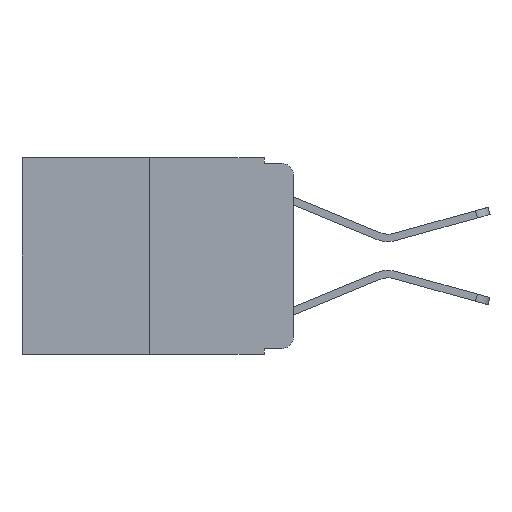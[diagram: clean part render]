
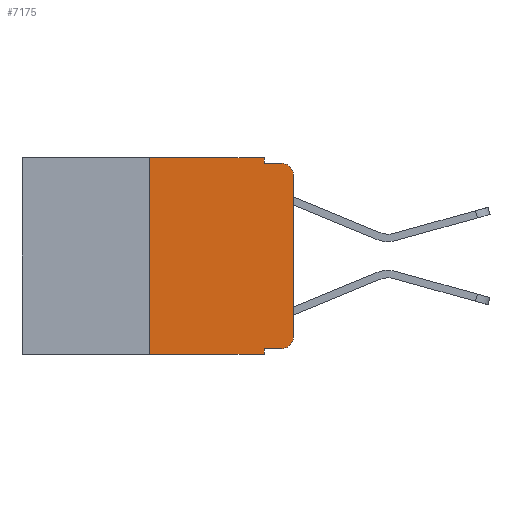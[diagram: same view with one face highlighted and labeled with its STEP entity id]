
A CAD part, left-side view. The second image highlights one B-rep face of the part: STEP entity #7175.
In plain terms, the highlighted planar face has unit normal (-1, 0, 0).
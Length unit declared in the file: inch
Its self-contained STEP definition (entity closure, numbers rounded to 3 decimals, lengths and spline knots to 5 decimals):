
#6 = EDGE_CURVE ( 'NONE', #13954, #5497, #19333, .T. ) ;
#8 = DIRECTION ( 'NONE',  ( 0., -1., 0. ) ) ;
#161 = EDGE_CURVE ( 'NONE', #24067, #17637, #10381, .T. ) ;
#260 = CARTESIAN_POINT ( 'NONE',  ( 0., 0.051, 0. ) ) ;
#411 = CARTESIAN_POINT ( 'NONE',  ( 0., 0.051, -0.333 ) ) ;
#908 = ORIENTED_EDGE ( 'NONE', *, *, #16106, .F. ) ;
#1094 = CARTESIAN_POINT ( 'NONE',  ( 0., 0.25, 0. ) ) ;
#1283 = CARTESIAN_POINT ( 'NONE',  ( 0., 0.051, -0.343 ) ) ;
#1460 = EDGE_CURVE ( 'NONE', #13954, #17637, #13989, .T. ) ;
#1534 = VERTEX_POINT ( 'NONE', #10384 ) ;
#2847 = DIRECTION ( 'NONE',  ( -1., 0., 0. ) ) ;
#2935 = VECTOR ( 'NONE', #17875, 39.37008 ) ;
#2961 = CARTESIAN_POINT ( 'NONE',  ( 0., 0., 0. ) ) ;
#3200 = ORIENTED_EDGE ( 'NONE', *, *, #1460, .T. ) ;
#3387 = CARTESIAN_POINT ( 'NONE',  ( 0., 0.02, -0.333 ) ) ;
#3432 = FACE_OUTER_BOUND ( 'NONE', #24683, .T. ) ;
#3738 = CARTESIAN_POINT ( 'NONE',  ( 0., 0.051, -0.333 ) ) ;
#3963 = ORIENTED_EDGE ( 'NONE', *, *, #21867, .T. ) ;
#4667 = CARTESIAN_POINT ( 'NONE',  ( 0., 0.051, -0.01 ) ) ;
#5497 = VERTEX_POINT ( 'NONE', #8939 ) ;
#5641 = AXIS2_PLACEMENT_3D ( 'NONE', #15857, #5842, #17981 ) ;
#5842 = DIRECTION ( 'NONE',  ( -1., 0., 0. ) ) ;
#6122 = ORIENTED_EDGE ( 'NONE', *, *, #25166, .T. ) ;
#6145 = CARTESIAN_POINT ( 'NONE',  ( 0., 0.25, -0.343 ) ) ;
#6511 = VERTEX_POINT ( 'NONE', #18292 ) ;
#7175 = ADVANCED_FACE ( 'NONE', ( #3432 ), #15705, .F. ) ;
#7245 = VECTOR ( 'NONE', #14246, 39.37008 ) ;
#7318 = VECTOR ( 'NONE', #8, 39.37008 ) ;
#7639 = VECTOR ( 'NONE', #11101, 39.37008 ) ;
#8404 = VERTEX_POINT ( 'NONE', #25243 ) ;
#8786 = VECTOR ( 'NONE', #16272, 39.37008 ) ;
#8939 = CARTESIAN_POINT ( 'NONE',  ( 0., 0.25, 0. ) ) ;
#9858 = DIRECTION ( 'NONE',  ( 0., 0., 1. ) ) ;
#9868 = LINE ( 'NONE', #3738, #2935 ) ;
#9883 = CIRCLE ( 'NONE', #5641, 0.02 ) ;
#10079 = ORIENTED_EDGE ( 'NONE', *, *, #14287, .T. ) ;
#10381 = LINE ( 'NONE', #260, #7245 ) ;
#10384 = CARTESIAN_POINT ( 'NONE',  ( 0., 0., -0.03 ) ) ;
#10443 = EDGE_CURVE ( 'NONE', #23450, #24132, #10587, .T. ) ;
#10571 = AXIS2_PLACEMENT_3D ( 'NONE', #25189, #2847, #23155 ) ;
#10587 = LINE ( 'NONE', #22868, #7639 ) ;
#10890 = CARTESIAN_POINT ( 'NONE',  ( 0., 0.051, -0.01 ) ) ;
#11101 = DIRECTION ( 'NONE',  ( 0., 0., -1. ) ) ;
#11247 = EDGE_CURVE ( 'NONE', #24132, #6511, #16786, .T. ) ;
#11900 = CARTESIAN_POINT ( 'NONE',  ( 0., 0.051, 0. ) ) ;
#12225 = ORIENTED_EDGE ( 'NONE', *, *, #11247, .F. ) ;
#12456 = CARTESIAN_POINT ( 'NONE',  ( 0., 0.473, 0. ) ) ;
#13289 = ORIENTED_EDGE ( 'NONE', *, *, #6, .F. ) ;
#13694 = CARTESIAN_POINT ( 'NONE',  ( 0., 0.473, 0. ) ) ;
#13954 = VERTEX_POINT ( 'NONE', #6145 ) ;
#13989 = LINE ( 'NONE', #24438, #7318 ) ;
#14246 = DIRECTION ( 'NONE',  ( 0., 0., -1. ) ) ;
#14287 = EDGE_CURVE ( 'NONE', #23400, #8404, #9883, .T. ) ;
#14651 = DIRECTION ( 'NONE',  ( 0., -1., 0. ) ) ;
#15705 = PLANE ( 'NONE',  #25161 ) ;
#15857 = CARTESIAN_POINT ( 'NONE',  ( 0., 0.02, -0.313 ) ) ;
#15949 = VECTOR ( 'NONE', #22480, 39.37008 ) ;
#16106 = EDGE_CURVE ( 'NONE', #5497, #23450, #18196, .T. ) ;
#16272 = DIRECTION ( 'NONE',  ( 0., 0., 1. ) ) ;
#16786 = LINE ( 'NONE', #10890, #18359 ) ;
#17637 = VERTEX_POINT ( 'NONE', #1283 ) ;
#17875 = DIRECTION ( 'NONE',  ( 0., -1., 0. ) ) ;
#17956 = ORIENTED_EDGE ( 'NONE', *, *, #23985, .T. ) ;
#17981 = DIRECTION ( 'NONE',  ( 0., 0., -1. ) ) ;
#18196 = LINE ( 'NONE', #12456, #15949 ) ;
#18292 = CARTESIAN_POINT ( 'NONE',  ( 0., 0.02, -0.01 ) ) ;
#18359 = VECTOR ( 'NONE', #14651, 39.37008 ) ;
#19333 = LINE ( 'NONE', #1094, #25193 ) ;
#19930 = CIRCLE ( 'NONE', #10571, 0.02 ) ;
#20477 = ORIENTED_EDGE ( 'NONE', *, *, #10443, .F. ) ;
#21221 = LINE ( 'NONE', #2961, #8786 ) ;
#21831 = DIRECTION ( 'NONE',  ( 1., 0., 0. ) ) ;
#21867 = EDGE_CURVE ( 'NONE', #1534, #6511, #19930, .T. ) ;
#22480 = DIRECTION ( 'NONE',  ( 0., -1., 0. ) ) ;
#22868 = CARTESIAN_POINT ( 'NONE',  ( 0., 0.051, 0. ) ) ;
#23155 = DIRECTION ( 'NONE',  ( 0., 0., -1. ) ) ;
#23400 = VERTEX_POINT ( 'NONE', #3387 ) ;
#23450 = VERTEX_POINT ( 'NONE', #11900 ) ;
#23985 = EDGE_CURVE ( 'NONE', #24067, #23400, #9868, .T. ) ;
#24005 = DIRECTION ( 'NONE',  ( 0., 0., -1. ) ) ;
#24067 = VERTEX_POINT ( 'NONE', #411 ) ;
#24132 = VERTEX_POINT ( 'NONE', #4667 ) ;
#24438 = CARTESIAN_POINT ( 'NONE',  ( 0., 0.473, -0.343 ) ) ;
#24683 = EDGE_LOOP ( 'NONE', ( #6122, #3963, #12225, #20477, #908, #13289, #3200, #25255, #17956, #10079 ) ) ;
#25161 = AXIS2_PLACEMENT_3D ( 'NONE', #13694, #21831, #24005 ) ;
#25166 = EDGE_CURVE ( 'NONE', #8404, #1534, #21221, .T. ) ;
#25189 = CARTESIAN_POINT ( 'NONE',  ( 0., 0.02, -0.03 ) ) ;
#25193 = VECTOR ( 'NONE', #9858, 39.37008 ) ;
#25243 = CARTESIAN_POINT ( 'NONE',  ( 0., 0., -0.313 ) ) ;
#25255 = ORIENTED_EDGE ( 'NONE', *, *, #161, .F. ) ;
